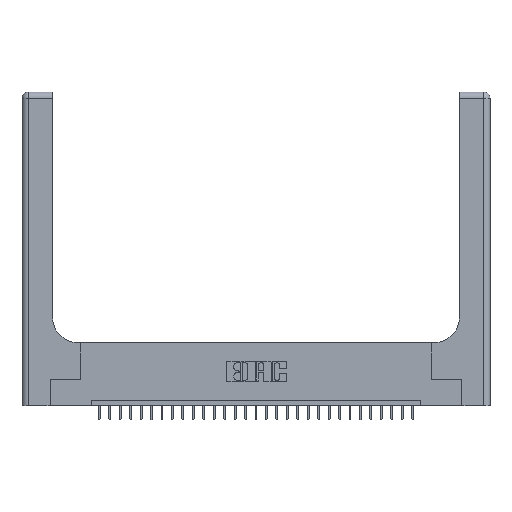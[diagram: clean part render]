
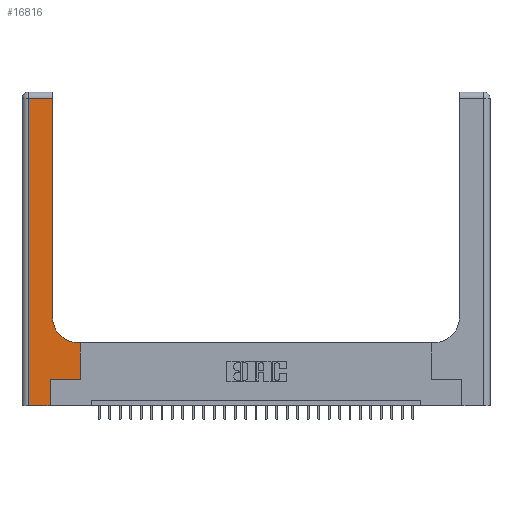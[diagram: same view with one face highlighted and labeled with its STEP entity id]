
A CAD part, top view. The second image highlights one B-rep face of the part: STEP entity #16816.
In plain terms, the highlighted planar face has unit normal (0, 0, 1).
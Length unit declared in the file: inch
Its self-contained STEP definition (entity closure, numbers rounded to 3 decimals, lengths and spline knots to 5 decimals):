
#1151 = VERTEX_POINT ( 'NONE', #11287 ) ;
#1389 = CARTESIAN_POINT ( 'NONE',  ( 0.2915, 0.6, 0.37 ) ) ;
#1498 = VECTOR ( 'NONE', #10231, 39.37008 ) ;
#1806 = LINE ( 'NONE', #6338, #9480 ) ;
#1900 = FACE_OUTER_BOUND ( 'NONE', #13263, .T. ) ;
#2121 = CARTESIAN_POINT ( 'NONE',  ( 0.5415, 0.6, 0.37 ) ) ;
#2429 = CARTESIAN_POINT ( 'NONE',  ( 0.269, 0., 0.37 ) ) ;
#4056 = DIRECTION ( 'NONE',  ( 0., 1., 0. ) ) ;
#4137 = VECTOR ( 'NONE', #4056, 39.37008 ) ;
#5175 = VECTOR ( 'NONE', #13244, 39.37008 ) ;
#5226 = DIRECTION ( 'NONE',  ( 0., -1., 0. ) ) ;
#5481 = EDGE_CURVE ( 'NONE', #20381, #20480, #12342, .T. ) ;
#5576 = CARTESIAN_POINT ( 'NONE',  ( 0.2915, 3., 0.37 ) ) ;
#6338 = CARTESIAN_POINT ( 'NONE',  ( 0., 2.94, 0.37 ) ) ;
#6552 = ORIENTED_EDGE ( 'NONE', *, *, #11787, .T. ) ;
#7150 = DIRECTION ( 'NONE',  ( 0., 0., -1. ) ) ;
#7176 = LINE ( 'NONE', #16491, #22113 ) ;
#7908 = CARTESIAN_POINT ( 'NONE',  ( 0.5585, 0.25, 0.37 ) ) ;
#8050 = LINE ( 'NONE', #1389, #17261 ) ;
#8217 = CARTESIAN_POINT ( 'NONE',  ( 0.2915, 2.94, 0.37 ) ) ;
#9480 = VECTOR ( 'NONE', #22032, 39.37008 ) ;
#9999 = AXIS2_PLACEMENT_3D ( 'NONE', #23478, #7150, #10055 ) ;
#10018 = CARTESIAN_POINT ( 'NONE',  ( 0.06, 0., 0.37 ) ) ;
#10055 = DIRECTION ( 'NONE',  ( 1., 0., 0. ) ) ;
#10231 = DIRECTION ( 'NONE',  ( 1., 0., 0. ) ) ;
#11159 = DIRECTION ( 'NONE',  ( -1., 0., 0. ) ) ;
#11287 = CARTESIAN_POINT ( 'NONE',  ( 0.2915, 0.85, 0.37 ) ) ;
#11787 = EDGE_CURVE ( 'NONE', #21210, #27058, #29341, .T. ) ;
#12342 = LINE ( 'NONE', #28931, #1498 ) ;
#12412 = ORIENTED_EDGE ( 'NONE', *, *, #17254, .T. ) ;
#12439 = VERTEX_POINT ( 'NONE', #15383 ) ;
#12750 = DIRECTION ( 'NONE',  ( 1., 0., 0. ) ) ;
#12990 = ORIENTED_EDGE ( 'NONE', *, *, #24235, .T. ) ;
#13046 = VERTEX_POINT ( 'NONE', #23433 ) ;
#13048 = LINE ( 'NONE', #29344, #4137 ) ;
#13244 = DIRECTION ( 'NONE',  ( 0., 1., 0. ) ) ;
#13263 = EDGE_LOOP ( 'NONE', ( #12990, #27614, #12412, #21833, #25905, #6552, #15088, #22116, #24660 ) ) ;
#14231 = VERTEX_POINT ( 'NONE', #8217 ) ;
#14842 = LINE ( 'NONE', #5576, #18213 ) ;
#15019 = CARTESIAN_POINT ( 'NONE',  ( 0.269, 0.25, 0.37 ) ) ;
#15059 = DIRECTION ( 'NONE',  ( -1., 0., 0. ) ) ;
#15088 = ORIENTED_EDGE ( 'NONE', *, *, #20134, .T. ) ;
#15383 = CARTESIAN_POINT ( 'NONE',  ( 0.06, 2.94, 0.37 ) ) ;
#15715 = DIRECTION ( 'NONE',  ( 0., 0., -1. ) ) ;
#16491 = CARTESIAN_POINT ( 'NONE',  ( 0.06, 3., 0.37 ) ) ;
#16816 = ADVANCED_FACE ( 'NONE', ( #1900 ), #26975, .F. ) ;
#17222 = AXIS2_PLACEMENT_3D ( 'NONE', #20473, #15715, #11159 ) ;
#17254 = EDGE_CURVE ( 'NONE', #12439, #20381, #7176, .T. ) ;
#17261 = VECTOR ( 'NONE', #15059, 39.37008 ) ;
#17887 = EDGE_CURVE ( 'NONE', #14231, #12439, #1806, .T. ) ;
#17902 = EDGE_CURVE ( 'NONE', #20480, #21210, #13048, .T. ) ;
#18213 = VECTOR ( 'NONE', #29180, 39.37008 ) ;
#19044 = EDGE_CURVE ( 'NONE', #13046, #23976, #8050, .T. ) ;
#20000 = EDGE_CURVE ( 'NONE', #23976, #1151, #23130, .T. ) ;
#20134 = EDGE_CURVE ( 'NONE', #27058, #13046, #29390, .T. ) ;
#20381 = VERTEX_POINT ( 'NONE', #10018 ) ;
#20396 = VECTOR ( 'NONE', #12750, 39.37008 ) ;
#20473 = CARTESIAN_POINT ( 'NONE',  ( 0., 3., 0.37 ) ) ;
#20480 = VERTEX_POINT ( 'NONE', #2429 ) ;
#21210 = VERTEX_POINT ( 'NONE', #28770 ) ;
#21746 = CARTESIAN_POINT ( 'NONE',  ( 0.5585, 0.25, 0.37 ) ) ;
#21833 = ORIENTED_EDGE ( 'NONE', *, *, #5481, .T. ) ;
#22032 = DIRECTION ( 'NONE',  ( -1., 0., 0. ) ) ;
#22113 = VECTOR ( 'NONE', #5226, 39.37008 ) ;
#22116 = ORIENTED_EDGE ( 'NONE', *, *, #19044, .T. ) ;
#23130 = CIRCLE ( 'NONE', #9999, 0.25 ) ;
#23433 = CARTESIAN_POINT ( 'NONE',  ( 0.5585, 0.6, 0.37 ) ) ;
#23478 = CARTESIAN_POINT ( 'NONE',  ( 0.5415, 0.85, 0.37 ) ) ;
#23976 = VERTEX_POINT ( 'NONE', #2121 ) ;
#24235 = EDGE_CURVE ( 'NONE', #1151, #14231, #14842, .T. ) ;
#24660 = ORIENTED_EDGE ( 'NONE', *, *, #20000, .T. ) ;
#25905 = ORIENTED_EDGE ( 'NONE', *, *, #17902, .T. ) ;
#26975 = PLANE ( 'NONE',  #17222 ) ;
#27058 = VERTEX_POINT ( 'NONE', #21746 ) ;
#27614 = ORIENTED_EDGE ( 'NONE', *, *, #17887, .T. ) ;
#28770 = CARTESIAN_POINT ( 'NONE',  ( 0.269, 0.25, 0.37 ) ) ;
#28931 = CARTESIAN_POINT ( 'NONE',  ( 0., 0., 0.37 ) ) ;
#29180 = DIRECTION ( 'NONE',  ( 0., 1., 0. ) ) ;
#29341 = LINE ( 'NONE', #15019, #20396 ) ;
#29344 = CARTESIAN_POINT ( 'NONE',  ( 0.269, 0., 0.37 ) ) ;
#29390 = LINE ( 'NONE', #7908, #5175 ) ;
